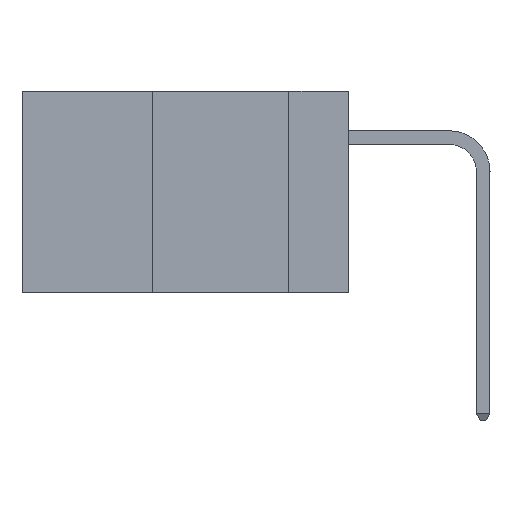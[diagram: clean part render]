
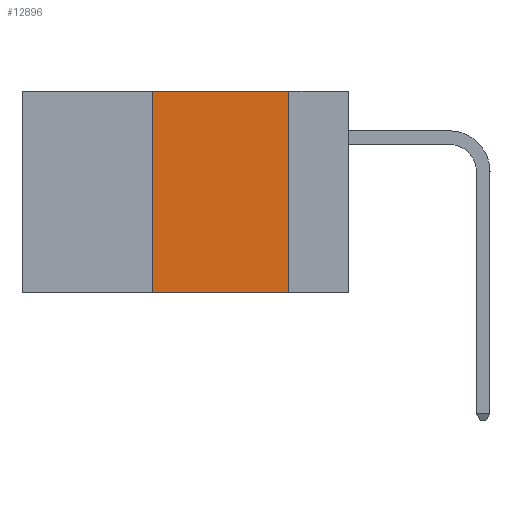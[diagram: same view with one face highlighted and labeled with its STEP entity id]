
A CAD part, left-side view. The second image highlights one B-rep face of the part: STEP entity #12896.
In plain terms, the highlighted planar face has unit normal (-1, 0, 0).
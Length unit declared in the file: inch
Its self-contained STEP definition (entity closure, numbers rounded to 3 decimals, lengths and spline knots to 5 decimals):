
#576 = CARTESIAN_POINT ( 'NONE',  ( 0., 0.6, 0. ) ) ;
#634 = EDGE_LOOP ( 'NONE', ( #22625, #8661, #24625, #30711 ) ) ;
#1329 = VECTOR ( 'NONE', #1396, 39.37008 ) ;
#1396 = DIRECTION ( 'NONE',  ( 0., 0., -1. ) ) ;
#5726 = VECTOR ( 'NONE', #26146, 39.37008 ) ;
#8661 = ORIENTED_EDGE ( 'NONE', *, *, #8907, .F. ) ;
#8907 = EDGE_CURVE ( 'NONE', #34440, #10385, #22322, .T. ) ;
#9193 = FACE_OUTER_BOUND ( 'NONE', #634, .T. ) ;
#10385 = VERTEX_POINT ( 'NONE', #28460 ) ;
#10457 = VECTOR ( 'NONE', #39027, 39.37008 ) ;
#12896 = ADVANCED_FACE ( 'NONE', ( #9193 ), #16445, .F. ) ;
#13854 = DIRECTION ( 'NONE',  ( 1., 0., 0. ) ) ;
#16445 = PLANE ( 'NONE',  #37674 ) ;
#16861 = CARTESIAN_POINT ( 'NONE',  ( 0., 0.11, 0. ) ) ;
#16879 = VERTEX_POINT ( 'NONE', #31993 ) ;
#16917 = VECTOR ( 'NONE', #24467, 39.37008 ) ;
#18032 = LINE ( 'NONE', #16861, #1329 ) ;
#20330 = LINE ( 'NONE', #27448, #16917 ) ;
#22322 = LINE ( 'NONE', #38550, #5726 ) ;
#22514 = CARTESIAN_POINT ( 'NONE',  ( 0., 0.11, -0.37 ) ) ;
#22625 = ORIENTED_EDGE ( 'NONE', *, *, #32375, .F. ) ;
#24467 = DIRECTION ( 'NONE',  ( 0., 0., 1. ) ) ;
#24625 = ORIENTED_EDGE ( 'NONE', *, *, #37537, .F. ) ;
#26146 = DIRECTION ( 'NONE',  ( 0., -1., 0. ) ) ;
#26326 = EDGE_CURVE ( 'NONE', #16879, #31613, #28097, .T. ) ;
#26360 = CARTESIAN_POINT ( 'NONE',  ( 0., 0.36, 0. ) ) ;
#27448 = CARTESIAN_POINT ( 'NONE',  ( 0., 0.36, 0. ) ) ;
#28097 = LINE ( 'NONE', #38769, #10457 ) ;
#28460 = CARTESIAN_POINT ( 'NONE',  ( 0., 0.11, 0. ) ) ;
#30200 = DIRECTION ( 'NONE',  ( 0., 0., -1. ) ) ;
#30711 = ORIENTED_EDGE ( 'NONE', *, *, #26326, .T. ) ;
#31613 = VERTEX_POINT ( 'NONE', #22514 ) ;
#31993 = CARTESIAN_POINT ( 'NONE',  ( 0., 0.36, -0.37 ) ) ;
#32375 = EDGE_CURVE ( 'NONE', #10385, #31613, #18032, .T. ) ;
#34440 = VERTEX_POINT ( 'NONE', #26360 ) ;
#37537 = EDGE_CURVE ( 'NONE', #16879, #34440, #20330, .T. ) ;
#37674 = AXIS2_PLACEMENT_3D ( 'NONE', #576, #13854, #30200 ) ;
#38550 = CARTESIAN_POINT ( 'NONE',  ( 0., 0.6, 0. ) ) ;
#38769 = CARTESIAN_POINT ( 'NONE',  ( 0., 0.6, -0.37 ) ) ;
#39027 = DIRECTION ( 'NONE',  ( 0., -1., 0. ) ) ;
